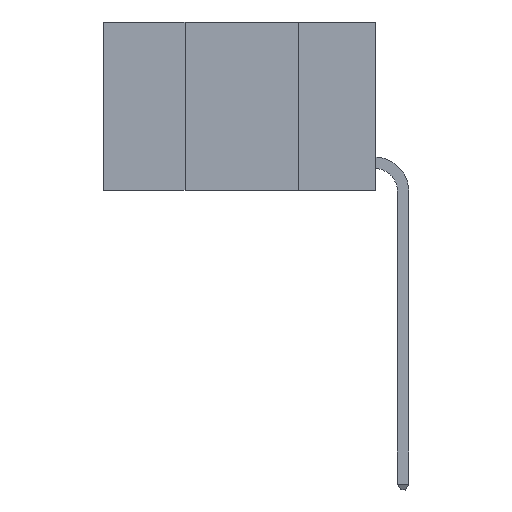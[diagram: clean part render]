
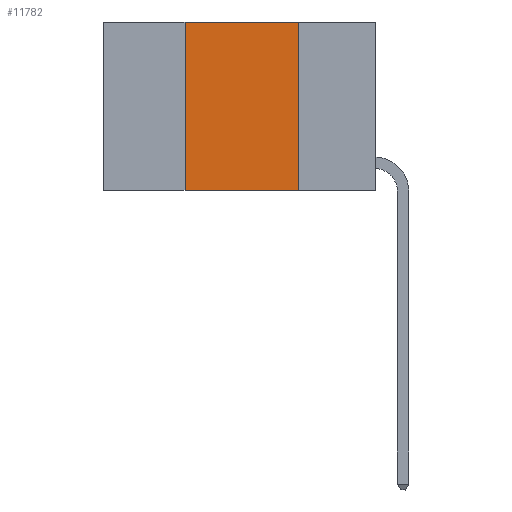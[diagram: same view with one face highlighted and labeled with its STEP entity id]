
A CAD part, left-side view. The second image highlights one B-rep face of the part: STEP entity #11782.
In plain terms, the highlighted planar face has unit normal (-1, 0, 0).
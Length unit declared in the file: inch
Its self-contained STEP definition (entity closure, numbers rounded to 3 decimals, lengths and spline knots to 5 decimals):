
#189 = VERTEX_POINT ( 'NONE', #24655 ) ;
#207 = LINE ( 'NONE', #6705, #12140 ) ;
#611 = CARTESIAN_POINT ( 'NONE',  ( 0., 0.42, 0. ) ) ;
#1805 = EDGE_CURVE ( 'NONE', #26391, #9178, #4196, .T. ) ;
#2816 = DIRECTION ( 'NONE',  ( 0., 0., -1. ) ) ;
#3067 = DIRECTION ( 'NONE',  ( 0., 0., 1. ) ) ;
#3176 = DIRECTION ( 'NONE',  ( 0., -1., 0. ) ) ;
#4196 = LINE ( 'NONE', #14098, #15164 ) ;
#5588 = EDGE_LOOP ( 'NONE', ( #28364, #22291, #20128, #24069 ) ) ;
#6196 = FACE_OUTER_BOUND ( 'NONE', #5588, .T. ) ;
#6705 = CARTESIAN_POINT ( 'NONE',  ( 0., 0.6, -0.37 ) ) ;
#6757 = CARTESIAN_POINT ( 'NONE',  ( 0., 0.6, 0. ) ) ;
#7024 = CARTESIAN_POINT ( 'NONE',  ( 0., 0.42, 0. ) ) ;
#7362 = EDGE_CURVE ( 'NONE', #9178, #25436, #8968, .T. ) ;
#8968 = LINE ( 'NONE', #19195, #25941 ) ;
#9053 = DIRECTION ( 'NONE',  ( 0., -1., 0. ) ) ;
#9116 = DIRECTION ( 'NONE',  ( 1., 0., 0. ) ) ;
#9178 = VERTEX_POINT ( 'NONE', #10863 ) ;
#10863 = CARTESIAN_POINT ( 'NONE',  ( 0., 0.17, 0. ) ) ;
#11088 = EDGE_CURVE ( 'NONE', #189, #25436, #207, .T. ) ;
#11782 = ADVANCED_FACE ( 'NONE', ( #6196 ), #20687, .F. ) ;
#12140 = VECTOR ( 'NONE', #9053, 39.37008 ) ;
#13072 = CARTESIAN_POINT ( 'NONE',  ( 0., 0.17, -0.37 ) ) ;
#14098 = CARTESIAN_POINT ( 'NONE',  ( 0., 0.6, 0. ) ) ;
#15164 = VECTOR ( 'NONE', #3176, 39.37008 ) ;
#17795 = AXIS2_PLACEMENT_3D ( 'NONE', #6757, #9116, #25264 ) ;
#18907 = LINE ( 'NONE', #611, #23566 ) ;
#19195 = CARTESIAN_POINT ( 'NONE',  ( 0., 0.17, 0. ) ) ;
#20128 = ORIENTED_EDGE ( 'NONE', *, *, #29564, .F. ) ;
#20687 = PLANE ( 'NONE',  #17795 ) ;
#22291 = ORIENTED_EDGE ( 'NONE', *, *, #1805, .F. ) ;
#23566 = VECTOR ( 'NONE', #3067, 39.37008 ) ;
#24069 = ORIENTED_EDGE ( 'NONE', *, *, #11088, .T. ) ;
#24655 = CARTESIAN_POINT ( 'NONE',  ( 0., 0.42, -0.37 ) ) ;
#25264 = DIRECTION ( 'NONE',  ( 0., 0., -1. ) ) ;
#25436 = VERTEX_POINT ( 'NONE', #13072 ) ;
#25941 = VECTOR ( 'NONE', #2816, 39.37008 ) ;
#26391 = VERTEX_POINT ( 'NONE', #7024 ) ;
#28364 = ORIENTED_EDGE ( 'NONE', *, *, #7362, .F. ) ;
#29564 = EDGE_CURVE ( 'NONE', #189, #26391, #18907, .T. ) ;
